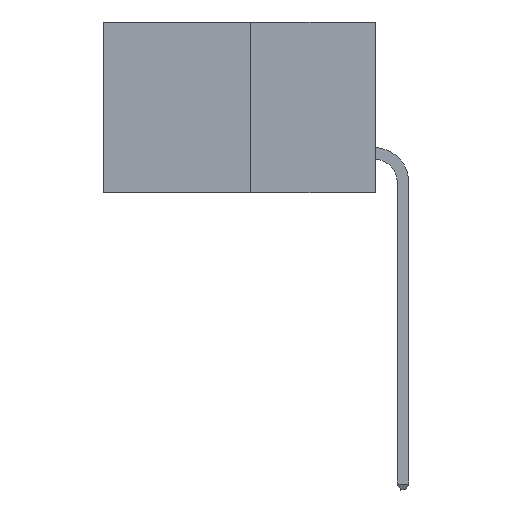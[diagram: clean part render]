
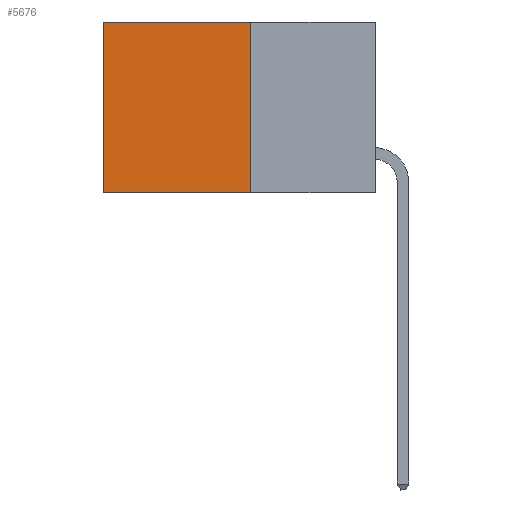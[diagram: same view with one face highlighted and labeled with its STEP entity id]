
A CAD part, left-side view. The second image highlights one B-rep face of the part: STEP entity #5676.
In plain terms, the highlighted planar face has unit normal (-1, 0, 0).
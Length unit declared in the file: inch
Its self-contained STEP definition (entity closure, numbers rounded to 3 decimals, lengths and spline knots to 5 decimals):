
#931 = VECTOR ( 'NONE', #7784, 39.37008 ) ;
#1195 = EDGE_CURVE ( 'NONE', #8699, #11210, #12838, .T. ) ;
#2130 = CARTESIAN_POINT ( 'NONE',  ( 0.277, 0.27, -0.37 ) ) ;
#2532 = AXIS2_PLACEMENT_3D ( 'NONE', #3690, #11548, #5721 ) ;
#2871 = CARTESIAN_POINT ( 'NONE',  ( 0.277, 0.59, -0.37 ) ) ;
#3234 = VECTOR ( 'NONE', #6851, 39.37008 ) ;
#3618 = LINE ( 'NONE', #5798, #931 ) ;
#3690 = CARTESIAN_POINT ( 'NONE',  ( 0.277, 0.27, -0.37 ) ) ;
#4257 = VECTOR ( 'NONE', #8900, 39.37008 ) ;
#4579 = CARTESIAN_POINT ( 'NONE',  ( 0.277, 0.59, 0. ) ) ;
#4921 = CARTESIAN_POINT ( 'NONE',  ( 0.277, 0.27, -0.37 ) ) ;
#4947 = VERTEX_POINT ( 'NONE', #4579 ) ;
#5676 = ADVANCED_FACE ( 'NONE', ( #11023 ), #10589, .F. ) ;
#5721 = DIRECTION ( 'NONE',  ( 0., 0., -1. ) ) ;
#5798 = CARTESIAN_POINT ( 'NONE',  ( 0.277, 0.27, 0. ) ) ;
#5847 = EDGE_CURVE ( 'NONE', #8778, #8699, #6915, .T. ) ;
#6851 = DIRECTION ( 'NONE',  ( 0., 0., -1. ) ) ;
#6915 = LINE ( 'NONE', #4921, #4257 ) ;
#7184 = ORIENTED_EDGE ( 'NONE', *, *, #1195, .F. ) ;
#7784 = DIRECTION ( 'NONE',  ( 0., 1., 0. ) ) ;
#8525 = EDGE_CURVE ( 'NONE', #4947, #11210, #11093, .T. ) ;
#8699 = VERTEX_POINT ( 'NONE', #2130 ) ;
#8778 = VERTEX_POINT ( 'NONE', #11092 ) ;
#8900 = DIRECTION ( 'NONE',  ( 0., 0., -1. ) ) ;
#10492 = CARTESIAN_POINT ( 'NONE',  ( 0.277, 0.59, -0.37 ) ) ;
#10589 = PLANE ( 'NONE',  #2532 ) ;
#10823 = EDGE_LOOP ( 'NONE', ( #12493, #7184, #12504, #11255 ) ) ;
#11023 = FACE_OUTER_BOUND ( 'NONE', #10823, .T. ) ;
#11092 = CARTESIAN_POINT ( 'NONE',  ( 0.277, 0.27, 0. ) ) ;
#11093 = LINE ( 'NONE', #2871, #3234 ) ;
#11210 = VERTEX_POINT ( 'NONE', #10492 ) ;
#11255 = ORIENTED_EDGE ( 'NONE', *, *, #12767, .T. ) ;
#11548 = DIRECTION ( 'NONE',  ( 1., 0., 0. ) ) ;
#12461 = DIRECTION ( 'NONE',  ( 0., 1., 0. ) ) ;
#12493 = ORIENTED_EDGE ( 'NONE', *, *, #8525, .T. ) ;
#12504 = ORIENTED_EDGE ( 'NONE', *, *, #5847, .F. ) ;
#12515 = VECTOR ( 'NONE', #12461, 39.37008 ) ;
#12659 = CARTESIAN_POINT ( 'NONE',  ( 0.277, 0.27, -0.37 ) ) ;
#12767 = EDGE_CURVE ( 'NONE', #8778, #4947, #3618, .T. ) ;
#12838 = LINE ( 'NONE', #12659, #12515 ) ;
